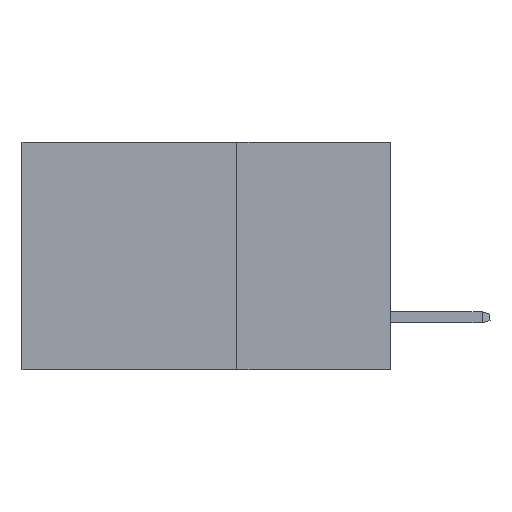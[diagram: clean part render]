
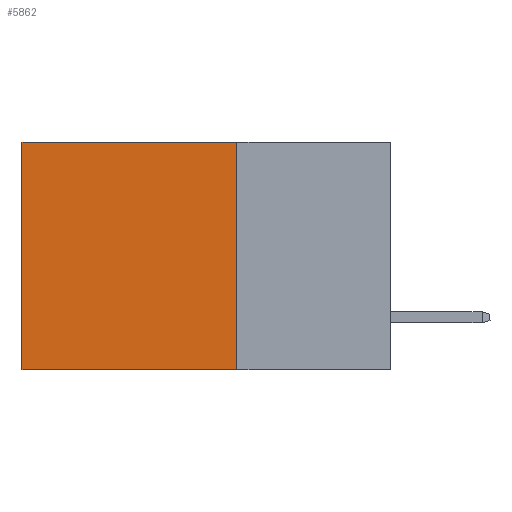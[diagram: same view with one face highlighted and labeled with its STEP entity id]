
A CAD part, left-side view. The second image highlights one B-rep face of the part: STEP entity #5862.
In plain terms, the highlighted planar face has unit normal (-1, 0, 0).
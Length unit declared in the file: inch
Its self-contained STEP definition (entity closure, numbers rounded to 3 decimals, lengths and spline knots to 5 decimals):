
#170 = VERTEX_POINT ( 'NONE', #4968 ) ;
#338 = FACE_OUTER_BOUND ( 'NONE', #8908, .T. ) ;
#643 = CARTESIAN_POINT ( 'NONE',  ( 0.2875, 0.25, 0. ) ) ;
#790 = DIRECTION ( 'NONE',  ( 0., 0., -1. ) ) ;
#1028 = CARTESIAN_POINT ( 'NONE',  ( 0.2875, 0.25, 0. ) ) ;
#1282 = VECTOR ( 'NONE', #5260, 39.37008 ) ;
#1387 = CARTESIAN_POINT ( 'NONE',  ( 0.2875, 0.25, 0. ) ) ;
#1623 = VERTEX_POINT ( 'NONE', #1028 ) ;
#2932 = CARTESIAN_POINT ( 'NONE',  ( 0.2875, 0.25, -0.37 ) ) ;
#3997 = DIRECTION ( 'NONE',  ( 1., 0., 0. ) ) ;
#4540 = VERTEX_POINT ( 'NONE', #2932 ) ;
#4968 = CARTESIAN_POINT ( 'NONE',  ( 0.2875, 0.6, -0.37 ) ) ;
#5116 = EDGE_CURVE ( 'NONE', #4540, #170, #5162, .T. ) ;
#5162 = LINE ( 'NONE', #10760, #5586 ) ;
#5243 = LINE ( 'NONE', #643, #5369 ) ;
#5260 = DIRECTION ( 'NONE',  ( 0., 1., 0. ) ) ;
#5369 = VECTOR ( 'NONE', #7544, 39.37008 ) ;
#5439 = CARTESIAN_POINT ( 'NONE',  ( 0.2875, 0.6, 0. ) ) ;
#5586 = VECTOR ( 'NONE', #9804, 39.37008 ) ;
#5805 = ORIENTED_EDGE ( 'NONE', *, *, #7983, .T. ) ;
#5862 = ADVANCED_FACE ( 'NONE', ( #338 ), #10868, .F. ) ;
#5906 = ORIENTED_EDGE ( 'NONE', *, *, #6198, .T. ) ;
#6198 = EDGE_CURVE ( 'NONE', #1623, #9534, #10541, .T. ) ;
#6364 = ORIENTED_EDGE ( 'NONE', *, *, #5116, .F. ) ;
#7455 = EDGE_CURVE ( 'NONE', #1623, #4540, #5243, .T. ) ;
#7492 = DIRECTION ( 'NONE',  ( 0., 0., -1. ) ) ;
#7544 = DIRECTION ( 'NONE',  ( 0., 0., -1. ) ) ;
#7983 = EDGE_CURVE ( 'NONE', #9534, #170, #9540, .T. ) ;
#8576 = VECTOR ( 'NONE', #790, 39.37008 ) ;
#8591 = CARTESIAN_POINT ( 'NONE',  ( 0.2875, 0.6, 0. ) ) ;
#8908 = EDGE_LOOP ( 'NONE', ( #5805, #6364, #9856, #5906 ) ) ;
#9534 = VERTEX_POINT ( 'NONE', #5439 ) ;
#9540 = LINE ( 'NONE', #8591, #8576 ) ;
#9804 = DIRECTION ( 'NONE',  ( 0., 1., 0. ) ) ;
#9856 = ORIENTED_EDGE ( 'NONE', *, *, #7455, .F. ) ;
#10504 = AXIS2_PLACEMENT_3D ( 'NONE', #1387, #3997, #7492 ) ;
#10541 = LINE ( 'NONE', #11233, #1282 ) ;
#10760 = CARTESIAN_POINT ( 'NONE',  ( 0.2875, 0.25, -0.37 ) ) ;
#10868 = PLANE ( 'NONE',  #10504 ) ;
#11233 = CARTESIAN_POINT ( 'NONE',  ( 0.2875, 0.25, 0. ) ) ;
